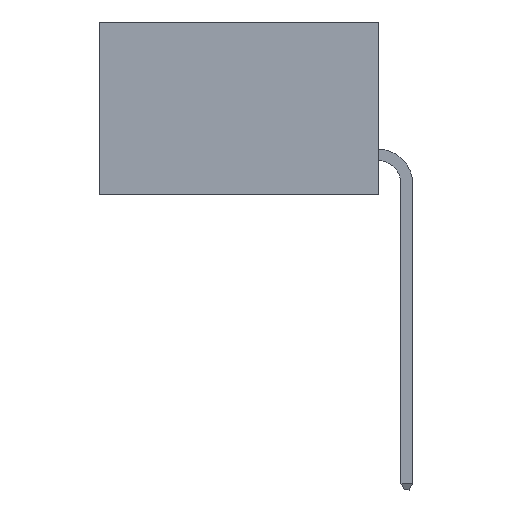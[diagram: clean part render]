
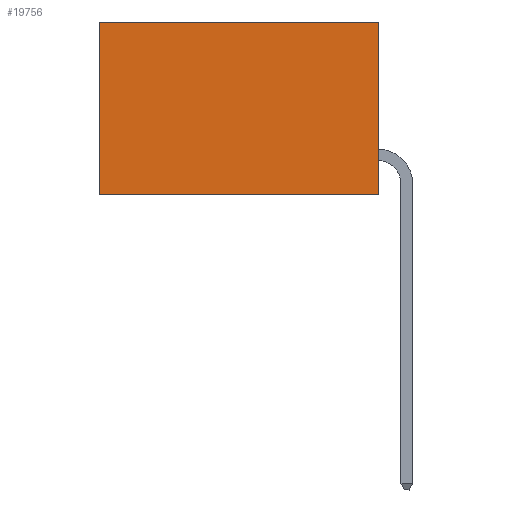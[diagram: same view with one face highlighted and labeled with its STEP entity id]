
A CAD part, left-side view. The second image highlights one B-rep face of the part: STEP entity #19756.
In plain terms, the highlighted planar face has unit normal (-1, 0, 0).
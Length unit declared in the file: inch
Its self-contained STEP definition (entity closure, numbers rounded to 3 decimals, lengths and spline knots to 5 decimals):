
#139 = CARTESIAN_POINT ( 'NONE',  ( 0.298, 0., 0. ) ) ;
#1401 = ORIENTED_EDGE ( 'NONE', *, *, #26083, .T. ) ;
#1556 = VERTEX_POINT ( 'NONE', #11077 ) ;
#2464 = DIRECTION ( 'NONE',  ( 0., 0., -1. ) ) ;
#2660 = ORIENTED_EDGE ( 'NONE', *, *, #31470, .F. ) ;
#4239 = EDGE_CURVE ( 'NONE', #6311, #1556, #14134, .T. ) ;
#4895 = ORIENTED_EDGE ( 'NONE', *, *, #19827, .T. ) ;
#6311 = VERTEX_POINT ( 'NONE', #18116 ) ;
#7404 = DIRECTION ( 'NONE',  ( 0., 0., -1. ) ) ;
#9207 = LINE ( 'NONE', #139, #27053 ) ;
#10751 = FACE_OUTER_BOUND ( 'NONE', #20815, .T. ) ;
#11077 = CARTESIAN_POINT ( 'NONE',  ( 0.298, 0.6, -0.37 ) ) ;
#11679 = CARTESIAN_POINT ( 'NONE',  ( 0.298, 0.6, 0. ) ) ;
#11862 = LINE ( 'NONE', #11679, #23977 ) ;
#11904 = VECTOR ( 'NONE', #7404, 39.37008 ) ;
#12595 = DIRECTION ( 'NONE',  ( 0., 1., 0. ) ) ;
#14134 = LINE ( 'NONE', #16207, #26229 ) ;
#16200 = CARTESIAN_POINT ( 'NONE',  ( 0.298, 0.6, 0. ) ) ;
#16207 = CARTESIAN_POINT ( 'NONE',  ( 0.298, 0., -0.37 ) ) ;
#17232 = DIRECTION ( 'NONE',  ( 1., 0., 0. ) ) ;
#17727 = VERTEX_POINT ( 'NONE', #16200 ) ;
#18116 = CARTESIAN_POINT ( 'NONE',  ( 0.298, 0., -0.37 ) ) ;
#18309 = CARTESIAN_POINT ( 'NONE',  ( 0.298, 0., 0. ) ) ;
#19067 = DIRECTION ( 'NONE',  ( 0., 0., -1. ) ) ;
#19756 = ADVANCED_FACE ( 'NONE', ( #10751 ), #29211, .F. ) ;
#19827 = EDGE_CURVE ( 'NONE', #28374, #17727, #9207, .T. ) ;
#20815 = EDGE_LOOP ( 'NONE', ( #1401, #23684, #2660, #4895 ) ) ;
#23240 = AXIS2_PLACEMENT_3D ( 'NONE', #31624, #17232, #2464 ) ;
#23684 = ORIENTED_EDGE ( 'NONE', *, *, #4239, .F. ) ;
#23977 = VECTOR ( 'NONE', #19067, 39.37008 ) ;
#24427 = CARTESIAN_POINT ( 'NONE',  ( 0.298, 0., 0. ) ) ;
#24792 = LINE ( 'NONE', #24427, #11904 ) ;
#25817 = DIRECTION ( 'NONE',  ( 0., 1., 0. ) ) ;
#26083 = EDGE_CURVE ( 'NONE', #17727, #1556, #11862, .T. ) ;
#26229 = VECTOR ( 'NONE', #25817, 39.37008 ) ;
#27053 = VECTOR ( 'NONE', #12595, 39.37008 ) ;
#28374 = VERTEX_POINT ( 'NONE', #18309 ) ;
#29211 = PLANE ( 'NONE',  #23240 ) ;
#31470 = EDGE_CURVE ( 'NONE', #28374, #6311, #24792, .T. ) ;
#31624 = CARTESIAN_POINT ( 'NONE',  ( 0.298, 0., 0. ) ) ;
